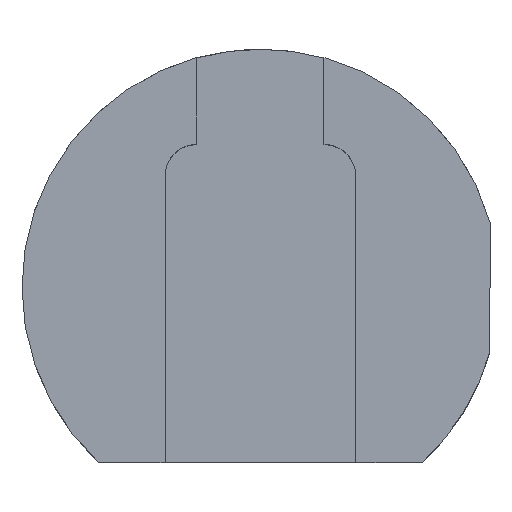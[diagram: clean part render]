
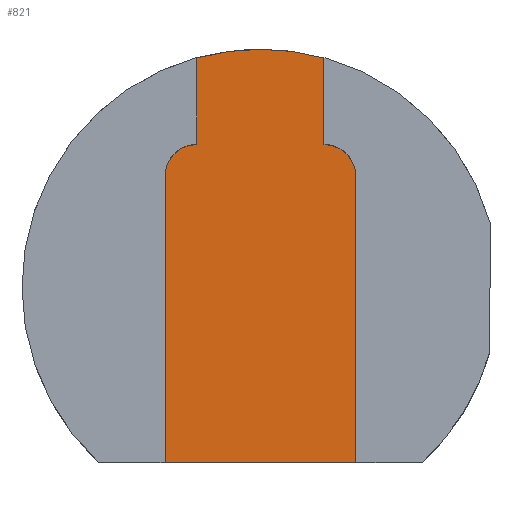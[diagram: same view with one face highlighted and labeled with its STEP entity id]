
A CAD part, top view. The second image highlights one B-rep face of the part: STEP entity #821.
In plain terms, the highlighted planar face has unit normal (0, 0, 1).
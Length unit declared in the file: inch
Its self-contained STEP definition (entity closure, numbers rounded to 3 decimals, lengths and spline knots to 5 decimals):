
#1 = ORIENTED_EDGE ( 'NONE', *, *, #421, .T. ) ;
#2 = DIRECTION ( 'NONE',  ( -1., 0., 0. ) ) ;
#19 = ORIENTED_EDGE ( 'NONE', *, *, #783, .T. ) ;
#30 = DIRECTION ( 'NONE',  ( 0., 0., -1. ) ) ;
#47 = EDGE_CURVE ( 'NONE', #326, #365, #311, .T. ) ;
#66 = EDGE_LOOP ( 'NONE', ( #19, #873, #579, #278, #706, #139, #435, #1 ) ) ;
#84 = AXIS2_PLACEMENT_3D ( 'NONE', #501, #30, #440 ) ;
#88 = CARTESIAN_POINT ( 'NONE',  ( -0.2, 0.9, -1.6 ) ) ;
#94 = CARTESIAN_POINT ( 'NONE',  ( -0.3, 0.35, -1.6 ) ) ;
#95 = VERTEX_POINT ( 'NONE', #722 ) ;
#109 = CARTESIAN_POINT ( 'NONE',  ( -0.2, 0.35, -1.6 ) ) ;
#125 = CARTESIAN_POINT ( 'NONE',  ( 0.2, 0.35, -1.6 ) ) ;
#131 = CARTESIAN_POINT ( 'NONE',  ( 0., 0., -1.6 ) ) ;
#139 = ORIENTED_EDGE ( 'NONE', *, *, #556, .T. ) ;
#146 = CIRCLE ( 'NONE', #780, 0.1 ) ;
#165 = DIRECTION ( 'NONE',  ( 0., -1., 0. ) ) ;
#169 = LINE ( 'NONE', #545, #422 ) ;
#178 = AXIS2_PLACEMENT_3D ( 'NONE', #131, #555, #266 ) ;
#190 = CARTESIAN_POINT ( 'NONE',  ( 0.3, -0.55, -1.6 ) ) ;
#202 = DIRECTION ( 'NONE',  ( 0., -1., 0. ) ) ;
#251 = DIRECTION ( 'NONE',  ( 0., -1., 0. ) ) ;
#253 = CIRCLE ( 'NONE', #517, 0.1 ) ;
#266 = DIRECTION ( 'NONE',  ( -1., 0., 0. ) ) ;
#278 = ORIENTED_EDGE ( 'NONE', *, *, #614, .F. ) ;
#290 = VECTOR ( 'NONE', #379, 39.37008 ) ;
#295 = VERTEX_POINT ( 'NONE', #94 ) ;
#296 = EDGE_CURVE ( 'NONE', #339, #477, #500, .T. ) ;
#303 = CARTESIAN_POINT ( 'NONE',  ( 0.3, 0.35, -1.6 ) ) ;
#309 = VECTOR ( 'NONE', #251, 39.37008 ) ;
#311 = LINE ( 'NONE', #548, #358 ) ;
#322 = LINE ( 'NONE', #88, #804 ) ;
#326 = VERTEX_POINT ( 'NONE', #303 ) ;
#339 = VERTEX_POINT ( 'NONE', #462 ) ;
#349 = VERTEX_POINT ( 'NONE', #524 ) ;
#358 = VECTOR ( 'NONE', #202, 39.37008 ) ;
#364 = LINE ( 'NONE', #599, #290 ) ;
#365 = VERTEX_POINT ( 'NONE', #190 ) ;
#379 = DIRECTION ( 'NONE',  ( 0., -1., 0. ) ) ;
#401 = EDGE_CURVE ( 'NONE', #349, #295, #146, .T. ) ;
#421 = EDGE_CURVE ( 'NONE', #295, #860, #885, .T. ) ;
#422 = VECTOR ( 'NONE', #697, 39.37008 ) ;
#435 = ORIENTED_EDGE ( 'NONE', *, *, #401, .T. ) ;
#440 = DIRECTION ( 'NONE',  ( -1., 0., 0. ) ) ;
#462 = CARTESIAN_POINT ( 'NONE',  ( -0.2, 0.72284, -1.6 ) ) ;
#473 = CARTESIAN_POINT ( 'NONE',  ( -0.3, -0.55, -1.6 ) ) ;
#477 = VERTEX_POINT ( 'NONE', #499 ) ;
#499 = CARTESIAN_POINT ( 'NONE',  ( 0.2, 0.72284, -1.6 ) ) ;
#500 = CIRCLE ( 'NONE', #84, 0.75 ) ;
#501 = CARTESIAN_POINT ( 'NONE',  ( 0., 0., -1.6 ) ) ;
#517 = AXIS2_PLACEMENT_3D ( 'NONE', #125, #896, #2 ) ;
#524 = CARTESIAN_POINT ( 'NONE',  ( -0.2, 0.45, -1.6 ) ) ;
#533 = DIRECTION ( 'NONE',  ( -1., 0., 0. ) ) ;
#545 = CARTESIAN_POINT ( 'NONE',  ( 0., -0.55, -1.6 ) ) ;
#548 = CARTESIAN_POINT ( 'NONE',  ( 0.3, 0., -1.6 ) ) ;
#555 = DIRECTION ( 'NONE',  ( 0., 0., -1. ) ) ;
#556 = EDGE_CURVE ( 'NONE', #339, #349, #322, .T. ) ;
#579 = ORIENTED_EDGE ( 'NONE', *, *, #645, .T. ) ;
#599 = CARTESIAN_POINT ( 'NONE',  ( 0.2, 0.9, -1.6 ) ) ;
#603 = CARTESIAN_POINT ( 'NONE',  ( -0.3, 0., -1.6 ) ) ;
#614 = EDGE_CURVE ( 'NONE', #477, #95, #364, .T. ) ;
#645 = EDGE_CURVE ( 'NONE', #326, #95, #253, .T. ) ;
#690 = PLANE ( 'NONE',  #178 ) ;
#697 = DIRECTION ( 'NONE',  ( 1., 0., 0. ) ) ;
#706 = ORIENTED_EDGE ( 'NONE', *, *, #296, .F. ) ;
#722 = CARTESIAN_POINT ( 'NONE',  ( 0.2, 0.45, -1.6 ) ) ;
#736 = DIRECTION ( 'NONE',  ( 0., 0., 1. ) ) ;
#780 = AXIS2_PLACEMENT_3D ( 'NONE', #109, #736, #533 ) ;
#783 = EDGE_CURVE ( 'NONE', #860, #365, #169, .T. ) ;
#786 = FACE_OUTER_BOUND ( 'NONE', #66, .T. ) ;
#804 = VECTOR ( 'NONE', #165, 39.37008 ) ;
#821 = ADVANCED_FACE ( 'NONE', ( #786 ), #690, .F. ) ;
#860 = VERTEX_POINT ( 'NONE', #473 ) ;
#873 = ORIENTED_EDGE ( 'NONE', *, *, #47, .F. ) ;
#885 = LINE ( 'NONE', #603, #309 ) ;
#896 = DIRECTION ( 'NONE',  ( 0., 0., 1. ) ) ;
